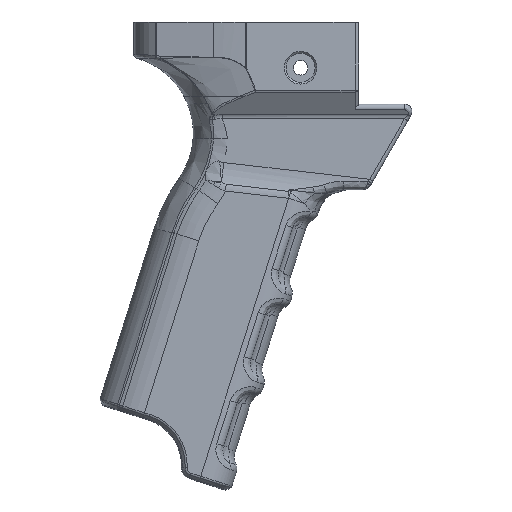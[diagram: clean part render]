
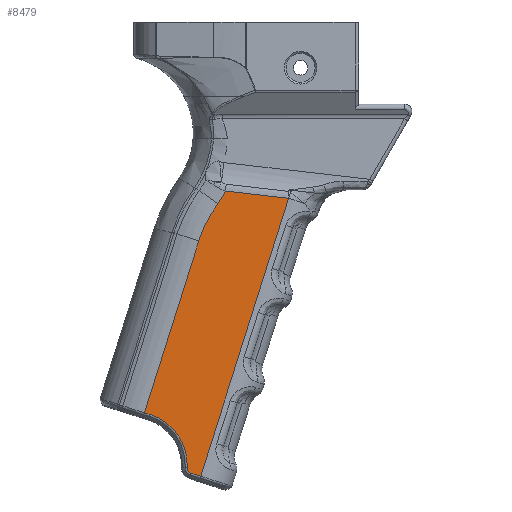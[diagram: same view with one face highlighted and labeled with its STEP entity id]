
A CAD part, front view. The second image highlights one B-rep face of the part: STEP entity #8479.
In plain terms, the highlighted planar face has unit normal (0, -1, 0).
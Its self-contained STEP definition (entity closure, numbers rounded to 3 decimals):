
#120=PLANE('',#9325);
#259=LINE('',#12389,#698);
#427=LINE('',#18044,#866);
#429=LINE('',#18062,#868);
#468=LINE('',#18691,#907);
#469=LINE('',#18696,#908);
#698=VECTOR('',#9788,10.);
#866=VECTOR('',#10848,10.);
#868=VECTOR('',#10870,10.);
#907=VECTOR('',#11107,10.);
#908=VECTOR('',#11112,10.);
#1423=B_SPLINE_CURVE_WITH_KNOTS('',3,(#18686,#18687,#18688,#18689),
 .UNSPECIFIED.,.F.,.F.,(4,4),(-0.018,0.),
 .UNSPECIFIED.);
#2016=FACE_OUTER_BOUND('',#2572,.T.);
#2572=EDGE_LOOP('',(#6851,#6852,#6853,#6854,#6855,#6856,#6857,#6858,#6859,
#6860));
#3114=CIRCLE('',#9220,1.419);
#3117=CIRCLE('',#9224,14.581);
#3171=CIRCLE('',#9326,34.246);
#3172=CIRCLE('',#9327,37.23);
#3401=VERTEX_POINT('',#12383);
#3402=VERTEX_POINT('',#12388);
#3749=VERTEX_POINT('',#18040);
#3751=VERTEX_POINT('',#18046);
#3753=VERTEX_POINT('',#18052);
#3755=VERTEX_POINT('',#18058);
#3810=VERTEX_POINT('',#18685);
#3811=VERTEX_POINT('',#18690);
#3812=VERTEX_POINT('',#18692);
#3813=VERTEX_POINT('',#18694);
#4177=EDGE_CURVE('',#3401,#3402,#259,.T.);
#4765=EDGE_CURVE('',#3402,#3749,#427,.T.);
#4768=EDGE_CURVE('',#3749,#3751,#3114,.T.);
#4771=EDGE_CURVE('',#3751,#3753,#3117,.T.);
#4774=EDGE_CURVE('',#3753,#3755,#429,.T.);
#4885=EDGE_CURVE('',#3810,#3401,#1423,.T.);
#4886=EDGE_CURVE('',#3811,#3810,#468,.T.);
#4887=EDGE_CURVE('',#3812,#3811,#3171,.T.);
#4888=EDGE_CURVE('',#3813,#3812,#3172,.T.);
#4889=EDGE_CURVE('',#3755,#3813,#469,.T.);
#6851=ORIENTED_EDGE('',*,*,#4765,.F.);
#6852=ORIENTED_EDGE('',*,*,#4177,.F.);
#6853=ORIENTED_EDGE('',*,*,#4885,.F.);
#6854=ORIENTED_EDGE('',*,*,#4886,.F.);
#6855=ORIENTED_EDGE('',*,*,#4887,.F.);
#6856=ORIENTED_EDGE('',*,*,#4888,.F.);
#6857=ORIENTED_EDGE('',*,*,#4889,.F.);
#6858=ORIENTED_EDGE('',*,*,#4774,.F.);
#6859=ORIENTED_EDGE('',*,*,#4771,.F.);
#6860=ORIENTED_EDGE('',*,*,#4768,.F.);
#8479=ADVANCED_FACE('',(#2016),#120,.T.);
#9220=AXIS2_PLACEMENT_3D('',#18050,#10855,#10856);
#9224=AXIS2_PLACEMENT_3D('',#18056,#10863,#10864);
#9325=AXIS2_PLACEMENT_3D('',#18684,#11105,#11106);
#9326=AXIS2_PLACEMENT_3D('',#18693,#11108,#11109);
#9327=AXIS2_PLACEMENT_3D('',#18695,#11110,#11111);
#9788=DIRECTION('',(-0.301,0.,-0.953));
#10848=DIRECTION('',(-0.953,0.,0.301));
#10855=DIRECTION('center_axis',(0.,1.,0.));
#10856=DIRECTION('ref_axis',(-0.822,0.,-0.569));
#10863=DIRECTION('center_axis',(0.,-1.,0.));
#10864=DIRECTION('ref_axis',(0.822,0.,0.569));
#10870=DIRECTION('',(-0.953,0.,0.301));
#11105=DIRECTION('center_axis',(0.,-1.,0.));
#11106=DIRECTION('ref_axis',(1.,0.,0.));
#11107=DIRECTION('',(0.993,0.,-0.114));
#11108=DIRECTION('center_axis',(0.,-1.,0.));
#11109=DIRECTION('ref_axis',(0.833,0.,-0.553));
#11110=DIRECTION('center_axis',(0.,1.,0.));
#11111=DIRECTION('ref_axis',(-0.888,0.,0.459));
#11112=DIRECTION('',(0.301,0.,0.953));
#12383=CARTESIAN_POINT('',(-154.447,3.068,-51.022));
#12388=CARTESIAN_POINT('',(-178.613,3.068,-127.473));
#12389=CARTESIAN_POINT('',(-158.165,3.068,-62.785));
#18040=CARTESIAN_POINT('',(-181.352,3.068,-126.607));
#18044=CARTESIAN_POINT('',(-176.104,3.068,-128.266));
#18046=CARTESIAN_POINT('',(-182.341,3.068,-125.178));
#18050=CARTESIAN_POINT('Origin',(-180.924,3.068,-125.254));
#18052=CARTESIAN_POINT('',(-192.507,3.068,-110.496));
#18056=CARTESIAN_POINT('Origin',(-196.901,3.068,-124.399));
#18058=CARTESIAN_POINT('',(-194.075,3.068,-110.));
#18062=CARTESIAN_POINT('',(-174.614,3.068,-116.151));
#18684=CARTESIAN_POINT('Origin',(-159.401,3.068,-74.198));
#18685=CARTESIAN_POINT('',(-154.624,3.068,-50.984));
#18686=CARTESIAN_POINT('Ctrl Pts',(-154.624,3.068,-50.984));
#18687=CARTESIAN_POINT('Ctrl Pts',(-154.564,3.068,-50.991));
#18688=CARTESIAN_POINT('Ctrl Pts',(-154.505,3.068,-51.003));
#18689=CARTESIAN_POINT('Ctrl Pts',(-154.447,3.068,-51.022));
#18690=CARTESIAN_POINT('',(-171.8,3.068,-49.012));
#18691=CARTESIAN_POINT('',(-144.123,3.068,-52.19));
#18692=CARTESIAN_POINT('',(-173.881,3.068,-52.467));
#18693=CARTESIAN_POINT('Origin',(-202.126,3.068,-33.103));
#18694=CARTESIAN_POINT('',(-179.14,3.068,-62.751));
#18695=CARTESIAN_POINT('Origin',(-143.765,3.068,-74.355));
#18696=CARTESIAN_POINT('',(-179.058,3.068,-62.491));
